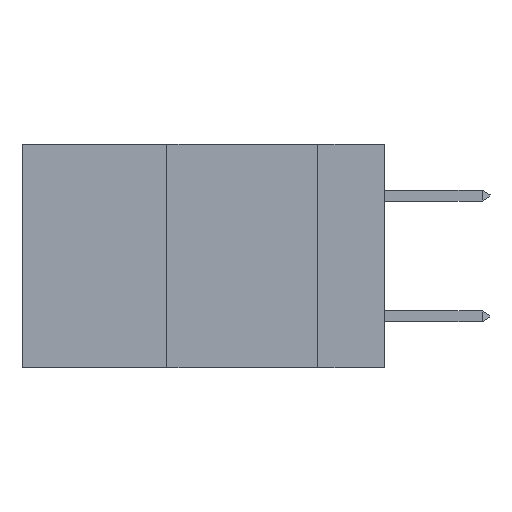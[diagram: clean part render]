
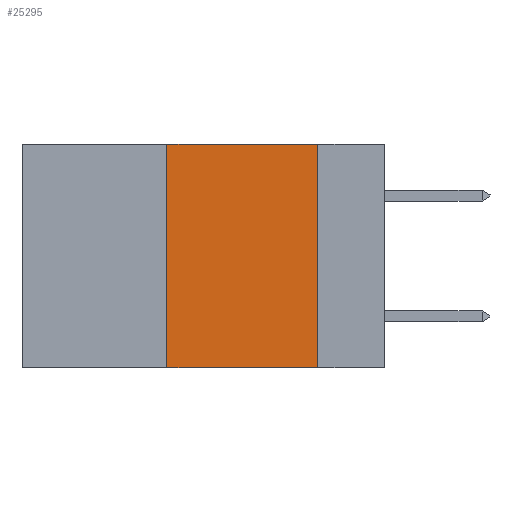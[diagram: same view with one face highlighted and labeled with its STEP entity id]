
A CAD part, left-side view. The second image highlights one B-rep face of the part: STEP entity #25295.
In plain terms, the highlighted planar face has unit normal (-1, 0, 0).
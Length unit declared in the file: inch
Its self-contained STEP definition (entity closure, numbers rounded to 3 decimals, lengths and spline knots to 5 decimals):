
#157 = AXIS2_PLACEMENT_3D ( 'NONE', #3567, #17535, #5578 ) ;
#211 = LINE ( 'NONE', #9437, #10160 ) ;
#1126 = VECTOR ( 'NONE', #19543, 39.37008 ) ;
#1554 = PLANE ( 'NONE',  #157 ) ;
#1990 = EDGE_CURVE ( 'NONE', #25666, #7195, #10076, .T. ) ;
#3567 = CARTESIAN_POINT ( 'NONE',  ( 0., 0.6, 0. ) ) ;
#3876 = CARTESIAN_POINT ( 'NONE',  ( 0., 0.36, 0. ) ) ;
#5578 = DIRECTION ( 'NONE',  ( 0., 0., -1. ) ) ;
#5675 = CARTESIAN_POINT ( 'NONE',  ( 0., 0.36, 0. ) ) ;
#6421 = LINE ( 'NONE', #15561, #1126 ) ;
#6847 = CARTESIAN_POINT ( 'NONE',  ( 0., 0.11, 0. ) ) ;
#7195 = VERTEX_POINT ( 'NONE', #21368 ) ;
#8778 = CARTESIAN_POINT ( 'NONE',  ( 0., 0.6, -0.37 ) ) ;
#9400 = ORIENTED_EDGE ( 'NONE', *, *, #23283, .F. ) ;
#9437 = CARTESIAN_POINT ( 'NONE',  ( 0., 0.6, 0. ) ) ;
#10076 = LINE ( 'NONE', #8778, #20169 ) ;
#10160 = VECTOR ( 'NONE', #21536, 39.37008 ) ;
#10801 = DIRECTION ( 'NONE',  ( 0., -1., 0. ) ) ;
#12562 = ORIENTED_EDGE ( 'NONE', *, *, #1990, .T. ) ;
#15140 = VECTOR ( 'NONE', #17843, 39.37008 ) ;
#15561 = CARTESIAN_POINT ( 'NONE',  ( 0., 0.11, 0. ) ) ;
#17535 = DIRECTION ( 'NONE',  ( 1., 0., 0. ) ) ;
#17843 = DIRECTION ( 'NONE',  ( 0., 0., 1. ) ) ;
#18099 = VERTEX_POINT ( 'NONE', #6847 ) ;
#18489 = EDGE_CURVE ( 'NONE', #20454, #18099, #211, .T. ) ;
#19374 = EDGE_LOOP ( 'NONE', ( #22238, #21683, #9400, #12562 ) ) ;
#19543 = DIRECTION ( 'NONE',  ( 0., 0., -1. ) ) ;
#20098 = FACE_OUTER_BOUND ( 'NONE', #19374, .T. ) ;
#20169 = VECTOR ( 'NONE', #10801, 39.37008 ) ;
#20454 = VERTEX_POINT ( 'NONE', #5675 ) ;
#21368 = CARTESIAN_POINT ( 'NONE',  ( 0., 0.11, -0.37 ) ) ;
#21536 = DIRECTION ( 'NONE',  ( 0., -1., 0. ) ) ;
#21683 = ORIENTED_EDGE ( 'NONE', *, *, #18489, .F. ) ;
#22238 = ORIENTED_EDGE ( 'NONE', *, *, #23197, .F. ) ;
#22738 = CARTESIAN_POINT ( 'NONE',  ( 0., 0.36, -0.37 ) ) ;
#23197 = EDGE_CURVE ( 'NONE', #18099, #7195, #6421, .T. ) ;
#23283 = EDGE_CURVE ( 'NONE', #25666, #20454, #24616, .T. ) ;
#24616 = LINE ( 'NONE', #3876, #15140 ) ;
#25295 = ADVANCED_FACE ( 'NONE', ( #20098 ), #1554, .F. ) ;
#25666 = VERTEX_POINT ( 'NONE', #22738 ) ;
